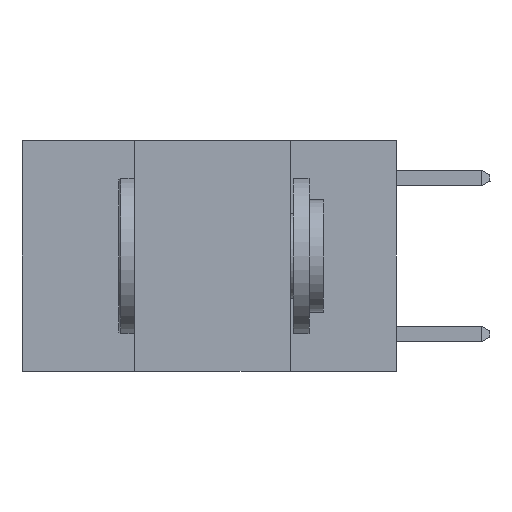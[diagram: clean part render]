
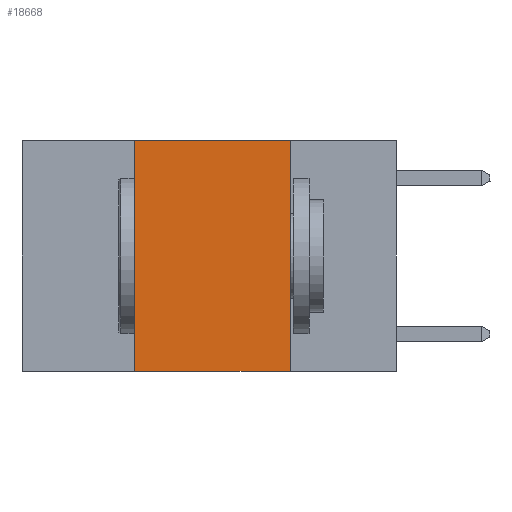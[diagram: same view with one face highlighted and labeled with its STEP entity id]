
A CAD part, left-side view. The second image highlights one B-rep face of the part: STEP entity #18668.
In plain terms, the highlighted planar face has unit normal (-1, 0, 0).
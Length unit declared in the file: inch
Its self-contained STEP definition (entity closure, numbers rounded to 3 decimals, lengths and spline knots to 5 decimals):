
#358 = EDGE_CURVE ( 'NONE', #17810, #4505, #6134, .T. ) ;
#1602 = CARTESIAN_POINT ( 'NONE',  ( 0., 0.42, 0. ) ) ;
#1900 = LINE ( 'NONE', #21165, #13651 ) ;
#2244 = EDGE_LOOP ( 'NONE', ( #17383, #9435, #27264, #24668 ) ) ;
#2483 = EDGE_CURVE ( 'NONE', #22695, #4505, #22037, .T. ) ;
#3075 = CARTESIAN_POINT ( 'NONE',  ( 0., 0.42, -0.37 ) ) ;
#3384 = DIRECTION ( 'NONE',  ( 0., -1., 0. ) ) ;
#3664 = LINE ( 'NONE', #1602, #7528 ) ;
#4505 = VERTEX_POINT ( 'NONE', #10420 ) ;
#6134 = LINE ( 'NONE', #23653, #16786 ) ;
#6214 = EDGE_CURVE ( 'NONE', #20545, #17810, #1900, .T. ) ;
#6747 = CARTESIAN_POINT ( 'NONE',  ( 0., 0.42, 0. ) ) ;
#7528 = VECTOR ( 'NONE', #13308, 39.37008 ) ;
#7806 = CARTESIAN_POINT ( 'NONE',  ( 0., 0.6, -0.37 ) ) ;
#9435 = ORIENTED_EDGE ( 'NONE', *, *, #6214, .F. ) ;
#10420 = CARTESIAN_POINT ( 'NONE',  ( 0., 0.17, -0.37 ) ) ;
#11338 = DIRECTION ( 'NONE',  ( 0., 0., -1. ) ) ;
#11862 = CARTESIAN_POINT ( 'NONE',  ( 0., 0.17, 0. ) ) ;
#12057 = FACE_OUTER_BOUND ( 'NONE', #2244, .T. ) ;
#13308 = DIRECTION ( 'NONE',  ( 0., 0., 1. ) ) ;
#13651 = VECTOR ( 'NONE', #30852, 39.37008 ) ;
#16786 = VECTOR ( 'NONE', #11338, 39.37008 ) ;
#17383 = ORIENTED_EDGE ( 'NONE', *, *, #358, .F. ) ;
#17810 = VERTEX_POINT ( 'NONE', #11862 ) ;
#18511 = VECTOR ( 'NONE', #3384, 39.37008 ) ;
#18668 = ADVANCED_FACE ( 'NONE', ( #12057 ), #26293, .F. ) ;
#20545 = VERTEX_POINT ( 'NONE', #6747 ) ;
#20949 = AXIS2_PLACEMENT_3D ( 'NONE', #29160, #22018, #24221 ) ;
#21165 = CARTESIAN_POINT ( 'NONE',  ( 0., 0.6, 0. ) ) ;
#21882 = EDGE_CURVE ( 'NONE', #22695, #20545, #3664, .T. ) ;
#22018 = DIRECTION ( 'NONE',  ( 1., 0., 0. ) ) ;
#22037 = LINE ( 'NONE', #7806, #18511 ) ;
#22695 = VERTEX_POINT ( 'NONE', #3075 ) ;
#23653 = CARTESIAN_POINT ( 'NONE',  ( 0., 0.17, 0. ) ) ;
#24221 = DIRECTION ( 'NONE',  ( 0., 0., -1. ) ) ;
#24668 = ORIENTED_EDGE ( 'NONE', *, *, #2483, .T. ) ;
#26293 = PLANE ( 'NONE',  #20949 ) ;
#27264 = ORIENTED_EDGE ( 'NONE', *, *, #21882, .F. ) ;
#29160 = CARTESIAN_POINT ( 'NONE',  ( 0., 0.6, 0. ) ) ;
#30852 = DIRECTION ( 'NONE',  ( 0., -1., 0. ) ) ;
